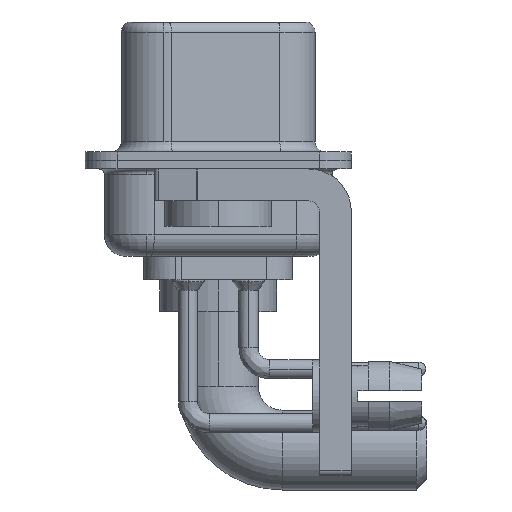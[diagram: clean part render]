
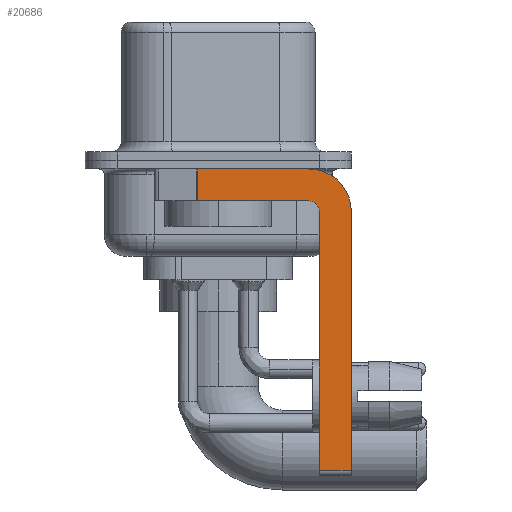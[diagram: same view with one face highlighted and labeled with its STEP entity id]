
A CAD part, left-side view. The second image highlights one B-rep face of the part: STEP entity #20686.
In plain terms, the highlighted planar face has unit normal (-1, 0, 0).
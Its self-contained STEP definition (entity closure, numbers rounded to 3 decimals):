
#34 = DIRECTION ( 'NONE',  ( 0., 0., -1. ) ) ;
#152 = VECTOR ( 'NONE', #14922, 1000. ) ;
#794 = VERTEX_POINT ( 'NONE', #5355 ) ;
#1046 = EDGE_CURVE ( 'NONE', #794, #10847, #17415, .T. ) ;
#1072 = DIRECTION ( 'NONE',  ( 0., 0., -1. ) ) ;
#1152 = AXIS2_PLACEMENT_3D ( 'NONE', #21334, #4223, #10568 ) ;
#1350 = CARTESIAN_POINT ( 'NONE',  ( -2.9, -6.25, -2.4 ) ) ;
#1385 = DIRECTION ( 'NONE',  ( 0., 0., -1. ) ) ;
#1925 = DIRECTION ( 'NONE',  ( 0., -1., 0. ) ) ;
#3721 = LINE ( 'NONE', #19523, #152 ) ;
#3938 = FACE_OUTER_BOUND ( 'NONE', #5594, .T. ) ;
#3950 = ORIENTED_EDGE ( 'NONE', *, *, #1046, .F. ) ;
#4223 = DIRECTION ( 'NONE',  ( -1., 0., 0. ) ) ;
#4743 = CARTESIAN_POINT ( 'NONE',  ( -2.9, 3., -0.4 ) ) ;
#5192 = VERTEX_POINT ( 'NONE', #26386 ) ;
#5355 = CARTESIAN_POINT ( 'NONE',  ( -2.9, 0.978, -0.4 ) ) ;
#5594 = EDGE_LOOP ( 'NONE', ( #3950, #8557, #7348, #14720, #21564, #10974, #25605, #11703 ) ) ;
#5999 = CARTESIAN_POINT ( 'NONE',  ( -2.9, -4.25, -2.4 ) ) ;
#6387 = DIRECTION ( 'NONE',  ( 1., 0., 0. ) ) ;
#6573 = CARTESIAN_POINT ( 'NONE',  ( -2.9, -4.75, -2.4 ) ) ;
#7312 = CARTESIAN_POINT ( 'NONE',  ( -2.9, -4.25, -0.4 ) ) ;
#7348 = ORIENTED_EDGE ( 'NONE', *, *, #20204, .F. ) ;
#7380 = DIRECTION ( 'NONE',  ( 0., 0., -1. ) ) ;
#7553 = AXIS2_PLACEMENT_3D ( 'NONE', #10976, #6387, #34 ) ;
#8557 = ORIENTED_EDGE ( 'NONE', *, *, #22280, .T. ) ;
#9928 = VECTOR ( 'NONE', #13502, 1000. ) ;
#9930 = EDGE_CURVE ( 'NONE', #27413, #5192, #12581, .T. ) ;
#10354 = CIRCLE ( 'NONE', #1152, 0.5 ) ;
#10568 = DIRECTION ( 'NONE',  ( 0., 0., 1. ) ) ;
#10847 = VERTEX_POINT ( 'NONE', #7312 ) ;
#10974 = ORIENTED_EDGE ( 'NONE', *, *, #9930, .T. ) ;
#10976 = CARTESIAN_POINT ( 'NONE',  ( -2.9, -4.25, -2.4 ) ) ;
#10987 = EDGE_CURVE ( 'NONE', #10847, #16791, #19111, .T. ) ;
#11703 = ORIENTED_EDGE ( 'NONE', *, *, #10987, .F. ) ;
#12581 = LINE ( 'NONE', #13138, #21527 ) ;
#13138 = CARTESIAN_POINT ( 'NONE',  ( -2.9, -4.25, -14.55 ) ) ;
#13502 = DIRECTION ( 'NONE',  ( 0., -1., 0. ) ) ;
#13772 = CARTESIAN_POINT ( 'NONE',  ( -2.9, -4.75, -14.55 ) ) ;
#14562 = CARTESIAN_POINT ( 'NONE',  ( -2.9, 0.978, -1.9 ) ) ;
#14720 = ORIENTED_EDGE ( 'NONE', *, *, #23980, .F. ) ;
#14785 = VERTEX_POINT ( 'NONE', #16357 ) ;
#14786 = DIRECTION ( 'NONE',  ( 0., 0., 1. ) ) ;
#14902 = VERTEX_POINT ( 'NONE', #6573 ) ;
#14922 = DIRECTION ( 'NONE',  ( 0., 1., 0. ) ) ;
#15067 = EDGE_CURVE ( 'NONE', #16791, #5192, #18767, .T. ) ;
#15134 = PLANE ( 'NONE',  #7553 ) ;
#15784 = VECTOR ( 'NONE', #7380, 1000. ) ;
#16357 = CARTESIAN_POINT ( 'NONE',  ( -2.9, -4.25, -1.9 ) ) ;
#16791 = VERTEX_POINT ( 'NONE', #1350 ) ;
#16813 = VERTEX_POINT ( 'NONE', #14562 ) ;
#17415 = LINE ( 'NONE', #4743, #9928 ) ;
#17510 = LINE ( 'NONE', #27897, #27430 ) ;
#17736 = AXIS2_PLACEMENT_3D ( 'NONE', #5999, #27706, #1385 ) ;
#18767 = LINE ( 'NONE', #27566, #28457 ) ;
#19111 = CIRCLE ( 'NONE', #17736, 2. ) ;
#19523 = CARTESIAN_POINT ( 'NONE',  ( -2.9, -4.25, -1.9 ) ) ;
#20204 = EDGE_CURVE ( 'NONE', #14785, #16813, #3721, .T. ) ;
#20686 = ADVANCED_FACE ( 'NONE', ( #3938 ), #15134, .F. ) ;
#21334 = CARTESIAN_POINT ( 'NONE',  ( -2.9, -4.25, -2.4 ) ) ;
#21527 = VECTOR ( 'NONE', #1925, 1000. ) ;
#21564 = ORIENTED_EDGE ( 'NONE', *, *, #27230, .F. ) ;
#22205 = LINE ( 'NONE', #22740, #15784 ) ;
#22280 = EDGE_CURVE ( 'NONE', #794, #16813, #22205, .T. ) ;
#22740 = CARTESIAN_POINT ( 'NONE',  ( -2.9, 0.978, -1.9 ) ) ;
#23980 = EDGE_CURVE ( 'NONE', #14902, #14785, #10354, .T. ) ;
#25605 = ORIENTED_EDGE ( 'NONE', *, *, #15067, .F. ) ;
#26386 = CARTESIAN_POINT ( 'NONE',  ( -2.9, -6.25, -14.55 ) ) ;
#27230 = EDGE_CURVE ( 'NONE', #27413, #14902, #17510, .T. ) ;
#27413 = VERTEX_POINT ( 'NONE', #13772 ) ;
#27430 = VECTOR ( 'NONE', #14786, 1000. ) ;
#27566 = CARTESIAN_POINT ( 'NONE',  ( -2.9, -6.25, -2.4 ) ) ;
#27706 = DIRECTION ( 'NONE',  ( 1., 0., 0. ) ) ;
#27897 = CARTESIAN_POINT ( 'NONE',  ( -2.9, -4.75, -14.8 ) ) ;
#28457 = VECTOR ( 'NONE', #1072, 1000. ) ;
